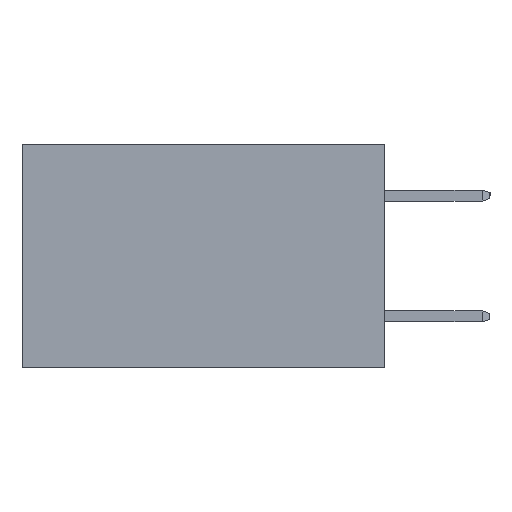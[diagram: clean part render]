
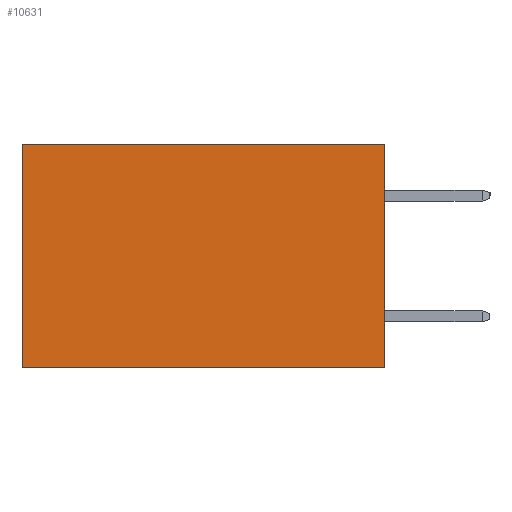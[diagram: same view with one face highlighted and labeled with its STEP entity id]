
A CAD part, left-side view. The second image highlights one B-rep face of the part: STEP entity #10631.
In plain terms, the highlighted planar face has unit normal (-1, 0, 0).
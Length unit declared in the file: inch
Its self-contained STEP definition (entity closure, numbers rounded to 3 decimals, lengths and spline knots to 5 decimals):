
#206 = ORIENTED_EDGE ( 'NONE', *, *, #10724, .T. ) ;
#1532 = PLANE ( 'NONE',  #3319 ) ;
#1920 = CARTESIAN_POINT ( 'NONE',  ( 0.2615, 0.6, 0. ) ) ;
#2074 = ORIENTED_EDGE ( 'NONE', *, *, #12084, .T. ) ;
#2324 = EDGE_CURVE ( 'NONE', #9102, #6145, #5796, .T. ) ;
#2547 = VERTEX_POINT ( 'NONE', #1920 ) ;
#2589 = CARTESIAN_POINT ( 'NONE',  ( 0.2615, 0., -0.37 ) ) ;
#2826 = FACE_OUTER_BOUND ( 'NONE', #4625, .T. ) ;
#3117 = LINE ( 'NONE', #4046, #9429 ) ;
#3193 = DIRECTION ( 'NONE',  ( 0., 0., -1. ) ) ;
#3319 = AXIS2_PLACEMENT_3D ( 'NONE', #2589, #7096, #12393 ) ;
#3569 = VECTOR ( 'NONE', #3193, 39.37008 ) ;
#3582 = VECTOR ( 'NONE', #3865, 39.37008 ) ;
#3865 = DIRECTION ( 'NONE',  ( 0., 0., -1. ) ) ;
#4046 = CARTESIAN_POINT ( 'NONE',  ( 0.2615, 0., 0. ) ) ;
#4371 = CARTESIAN_POINT ( 'NONE',  ( 0.2615, 0.6, -0.37 ) ) ;
#4392 = DIRECTION ( 'NONE',  ( 0., 1., 0. ) ) ;
#4625 = EDGE_LOOP ( 'NONE', ( #2074, #5826, #6962, #206 ) ) ;
#4926 = CARTESIAN_POINT ( 'NONE',  ( 0.2615, 0., -0.37 ) ) ;
#5328 = CARTESIAN_POINT ( 'NONE',  ( 0.2615, 0., -0.37 ) ) ;
#5678 = CARTESIAN_POINT ( 'NONE',  ( 0.2615, 0., 0. ) ) ;
#5796 = LINE ( 'NONE', #5328, #11295 ) ;
#5826 = ORIENTED_EDGE ( 'NONE', *, *, #2324, .F. ) ;
#5936 = LINE ( 'NONE', #4926, #3582 ) ;
#6145 = VERTEX_POINT ( 'NONE', #4371 ) ;
#6962 = ORIENTED_EDGE ( 'NONE', *, *, #12880, .F. ) ;
#7096 = DIRECTION ( 'NONE',  ( 1., 0., 0. ) ) ;
#9102 = VERTEX_POINT ( 'NONE', #9205 ) ;
#9205 = CARTESIAN_POINT ( 'NONE',  ( 0.2615, 0., -0.37 ) ) ;
#9429 = VECTOR ( 'NONE', #12939, 39.37008 ) ;
#9557 = LINE ( 'NONE', #9621, #3569 ) ;
#9621 = CARTESIAN_POINT ( 'NONE',  ( 0.2615, 0.6, -0.37 ) ) ;
#10414 = VERTEX_POINT ( 'NONE', #5678 ) ;
#10631 = ADVANCED_FACE ( 'NONE', ( #2826 ), #1532, .F. ) ;
#10724 = EDGE_CURVE ( 'NONE', #10414, #2547, #3117, .T. ) ;
#11295 = VECTOR ( 'NONE', #4392, 39.37008 ) ;
#12084 = EDGE_CURVE ( 'NONE', #2547, #6145, #9557, .T. ) ;
#12393 = DIRECTION ( 'NONE',  ( 0., 0., -1. ) ) ;
#12880 = EDGE_CURVE ( 'NONE', #10414, #9102, #5936, .T. ) ;
#12939 = DIRECTION ( 'NONE',  ( 0., 1., 0. ) ) ;
